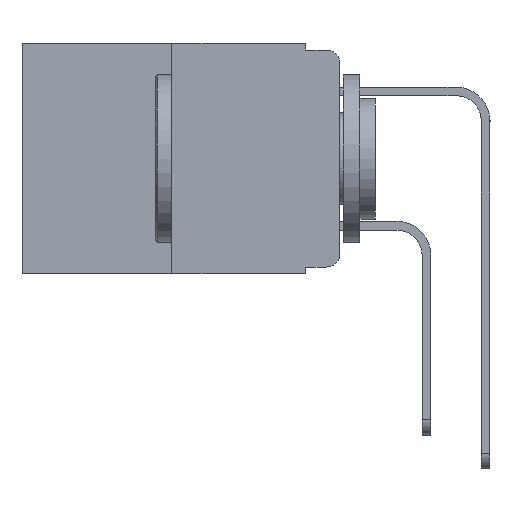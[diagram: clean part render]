
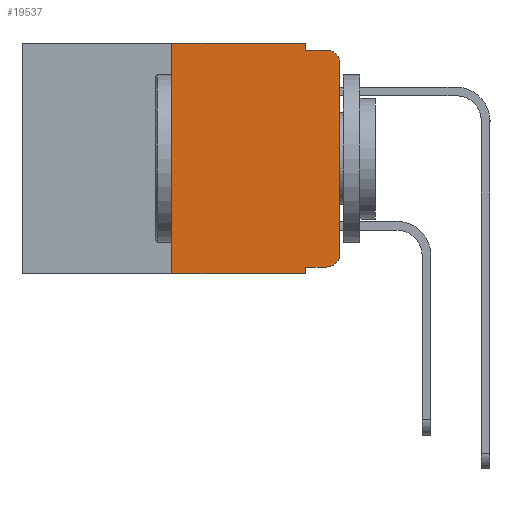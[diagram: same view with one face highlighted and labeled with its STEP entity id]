
A CAD part, left-side view. The second image highlights one B-rep face of the part: STEP entity #19537.
In plain terms, the highlighted planar face has unit normal (-1, 0, 0).
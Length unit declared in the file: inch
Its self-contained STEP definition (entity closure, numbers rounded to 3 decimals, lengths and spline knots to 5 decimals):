
#244 = DIRECTION ( 'NONE',  ( 1., 0., 0. ) ) ;
#253 = CARTESIAN_POINT ( 'NONE',  ( 0., 0.02, -0.01 ) ) ;
#343 = VECTOR ( 'NONE', #18559, 39.37008 ) ;
#770 = LINE ( 'NONE', #5712, #10539 ) ;
#971 = ORIENTED_EDGE ( 'NONE', *, *, #13671, .T. ) ;
#1717 = CARTESIAN_POINT ( 'NONE',  ( 0., 0.02, -0.333 ) ) ;
#1957 = EDGE_CURVE ( 'NONE', #17015, #18847, #19081, .T. ) ;
#2365 = DIRECTION ( 'NONE',  ( 0., -1., 0. ) ) ;
#3053 = VERTEX_POINT ( 'NONE', #17897 ) ;
#3828 = ORIENTED_EDGE ( 'NONE', *, *, #16980, .F. ) ;
#4147 = VECTOR ( 'NONE', #16341, 39.37008 ) ;
#4476 = VERTEX_POINT ( 'NONE', #23795 ) ;
#4709 = EDGE_CURVE ( 'NONE', #5707, #9101, #19542, .T. ) ;
#5581 = VECTOR ( 'NONE', #14390, 39.37008 ) ;
#5678 = LINE ( 'NONE', #16639, #343 ) ;
#5707 = VERTEX_POINT ( 'NONE', #18015 ) ;
#5712 = CARTESIAN_POINT ( 'NONE',  ( 0., 0., 0. ) ) ;
#6176 = LINE ( 'NONE', #18209, #5581 ) ;
#6694 = VECTOR ( 'NONE', #24689, 39.37008 ) ;
#6821 = CARTESIAN_POINT ( 'NONE',  ( 0., 0.051, -0.01 ) ) ;
#6908 = EDGE_CURVE ( 'NONE', #9850, #20449, #15891, .T. ) ;
#6975 = CARTESIAN_POINT ( 'NONE',  ( 0., 0.02, -0.03 ) ) ;
#8148 = AXIS2_PLACEMENT_3D ( 'NONE', #6975, #20298, #8901 ) ;
#8482 = LINE ( 'NONE', #13348, #6694 ) ;
#8683 = CARTESIAN_POINT ( 'NONE',  ( 0., 0.051, -0.01 ) ) ;
#8901 = DIRECTION ( 'NONE',  ( 0., 0., -1. ) ) ;
#9101 = VERTEX_POINT ( 'NONE', #6821 ) ;
#9219 = VECTOR ( 'NONE', #14015, 39.37008 ) ;
#9222 = LINE ( 'NONE', #8683, #4147 ) ;
#9621 = CARTESIAN_POINT ( 'NONE',  ( 0., 0.02, -0.313 ) ) ;
#9850 = VERTEX_POINT ( 'NONE', #18450 ) ;
#10539 = VECTOR ( 'NONE', #13284, 39.37008 ) ;
#10956 = EDGE_CURVE ( 'NONE', #21668, #3053, #5678, .T. ) ;
#11531 = DIRECTION ( 'NONE',  ( 0., 0., -1. ) ) ;
#12000 = CARTESIAN_POINT ( 'NONE',  ( 0., 0., -0.313 ) ) ;
#12092 = CARTESIAN_POINT ( 'NONE',  ( 0., 0.473, 0. ) ) ;
#12499 = ORIENTED_EDGE ( 'NONE', *, *, #1957, .T. ) ;
#12706 = EDGE_CURVE ( 'NONE', #17015, #4476, #6176, .T. ) ;
#13051 = EDGE_LOOP ( 'NONE', ( #17854, #23489, #3828, #14594, #24653, #15777, #971, #16966, #12499, #23207 ) ) ;
#13082 = DIRECTION ( 'NONE',  ( 0., 0., -1. ) ) ;
#13284 = DIRECTION ( 'NONE',  ( 0., 0., 1. ) ) ;
#13348 = CARTESIAN_POINT ( 'NONE',  ( 0., 0.473, -0.343 ) ) ;
#13671 = EDGE_CURVE ( 'NONE', #21668, #4476, #8482, .T. ) ;
#13846 = DIRECTION ( 'NONE',  ( 0., 0., -1. ) ) ;
#13874 = VERTEX_POINT ( 'NONE', #12000 ) ;
#13888 = VECTOR ( 'NONE', #13082, 39.37008 ) ;
#14015 = DIRECTION ( 'NONE',  ( 0., -1., 0. ) ) ;
#14024 = VECTOR ( 'NONE', #2365, 39.37008 ) ;
#14390 = DIRECTION ( 'NONE',  ( 0., 0., -1. ) ) ;
#14594 = ORIENTED_EDGE ( 'NONE', *, *, #4709, .F. ) ;
#14728 = EDGE_CURVE ( 'NONE', #13874, #9850, #770, .T. ) ;
#15669 = CARTESIAN_POINT ( 'NONE',  ( 0., 0.473, 0. ) ) ;
#15777 = ORIENTED_EDGE ( 'NONE', *, *, #10956, .F. ) ;
#15891 = CIRCLE ( 'NONE', #8148, 0.02 ) ;
#16341 = DIRECTION ( 'NONE',  ( 0., -1., 0. ) ) ;
#16639 = CARTESIAN_POINT ( 'NONE',  ( 0., 0.25, 0. ) ) ;
#16863 = FACE_OUTER_BOUND ( 'NONE', #13051, .T. ) ;
#16966 = ORIENTED_EDGE ( 'NONE', *, *, #12706, .F. ) ;
#16980 = EDGE_CURVE ( 'NONE', #9101, #20449, #9222, .T. ) ;
#17015 = VERTEX_POINT ( 'NONE', #20262 ) ;
#17854 = ORIENTED_EDGE ( 'NONE', *, *, #14728, .T. ) ;
#17897 = CARTESIAN_POINT ( 'NONE',  ( 0., 0.25, 0. ) ) ;
#18015 = CARTESIAN_POINT ( 'NONE',  ( 0., 0.051, 0. ) ) ;
#18117 = CARTESIAN_POINT ( 'NONE',  ( 0., 0.051, -0.333 ) ) ;
#18209 = CARTESIAN_POINT ( 'NONE',  ( 0., 0.051, 0. ) ) ;
#18450 = CARTESIAN_POINT ( 'NONE',  ( 0., 0., -0.03 ) ) ;
#18559 = DIRECTION ( 'NONE',  ( 0., 0., 1. ) ) ;
#18725 = CARTESIAN_POINT ( 'NONE',  ( 0., 0.051, 0. ) ) ;
#18847 = VERTEX_POINT ( 'NONE', #1717 ) ;
#19002 = LINE ( 'NONE', #12092, #9219 ) ;
#19081 = LINE ( 'NONE', #18117, #14024 ) ;
#19496 = PLANE ( 'NONE',  #21310 ) ;
#19537 = ADVANCED_FACE ( 'NONE', ( #16863 ), #19496, .F. ) ;
#19542 = LINE ( 'NONE', #18725, #13888 ) ;
#20262 = CARTESIAN_POINT ( 'NONE',  ( 0., 0.051, -0.333 ) ) ;
#20298 = DIRECTION ( 'NONE',  ( -1., 0., 0. ) ) ;
#20449 = VERTEX_POINT ( 'NONE', #253 ) ;
#20503 = EDGE_CURVE ( 'NONE', #3053, #5707, #19002, .T. ) ;
#20883 = CARTESIAN_POINT ( 'NONE',  ( 0., 0.25, -0.343 ) ) ;
#21310 = AXIS2_PLACEMENT_3D ( 'NONE', #15669, #244, #13846 ) ;
#21668 = VERTEX_POINT ( 'NONE', #20883 ) ;
#22132 = AXIS2_PLACEMENT_3D ( 'NONE', #9621, #22932, #11531 ) ;
#22319 = EDGE_CURVE ( 'NONE', #18847, #13874, #22501, .T. ) ;
#22501 = CIRCLE ( 'NONE', #22132, 0.02 ) ;
#22932 = DIRECTION ( 'NONE',  ( -1., 0., 0. ) ) ;
#23207 = ORIENTED_EDGE ( 'NONE', *, *, #22319, .T. ) ;
#23489 = ORIENTED_EDGE ( 'NONE', *, *, #6908, .T. ) ;
#23795 = CARTESIAN_POINT ( 'NONE',  ( 0., 0.051, -0.343 ) ) ;
#24653 = ORIENTED_EDGE ( 'NONE', *, *, #20503, .F. ) ;
#24689 = DIRECTION ( 'NONE',  ( 0., -1., 0. ) ) ;
